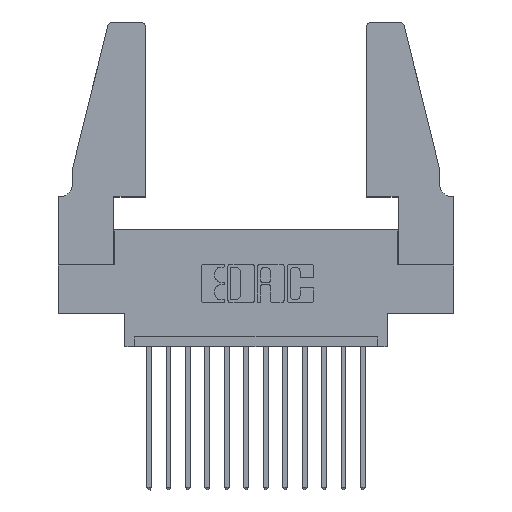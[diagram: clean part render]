
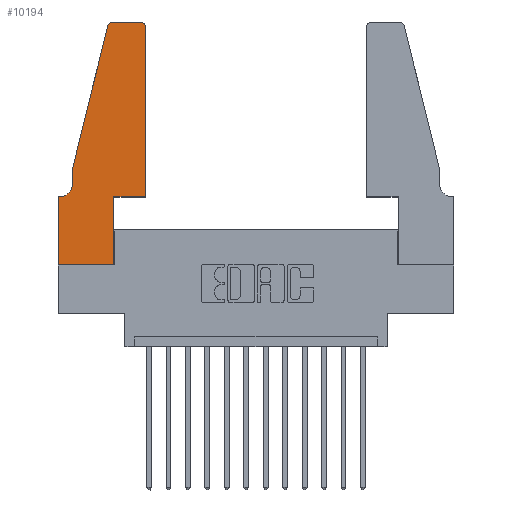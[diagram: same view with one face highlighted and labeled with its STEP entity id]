
A CAD part, top view. The second image highlights one B-rep face of the part: STEP entity #10194.
In plain terms, the highlighted planar face has unit normal (0, 0, 1).
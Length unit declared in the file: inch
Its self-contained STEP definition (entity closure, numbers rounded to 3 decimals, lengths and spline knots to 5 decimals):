
#111 = CARTESIAN_POINT ( 'NONE',  ( 0., 0.35, 0.37 ) ) ;
#120 = ORIENTED_EDGE ( 'NONE', *, *, #9475, .T. ) ;
#334 = CARTESIAN_POINT ( 'NONE',  ( 0., 0.35, 0.37 ) ) ;
#475 = VECTOR ( 'NONE', #14309, 39.37008 ) ;
#499 = EDGE_CURVE ( 'NONE', #13492, #5535, #6857, .T. ) ;
#622 = DIRECTION ( 'NONE',  ( -1., 0., 0. ) ) ;
#713 = DIRECTION ( 'NONE',  ( 1., 0., 0. ) ) ;
#787 = DIRECTION ( 'NONE',  ( 0., 0., -1. ) ) ;
#894 = VERTEX_POINT ( 'NONE', #9341 ) ;
#969 = VERTEX_POINT ( 'NONE', #13915 ) ;
#1103 = DIRECTION ( 'NONE',  ( 0., -1., 0. ) ) ;
#1887 = CARTESIAN_POINT ( 'NONE',  ( 0., 0., 0.37 ) ) ;
#2113 = EDGE_CURVE ( 'NONE', #12750, #4990, #7534, .T. ) ;
#2350 = EDGE_CURVE ( 'NONE', #4990, #13492, #3491, .T. ) ;
#2622 = CIRCLE ( 'NONE', #11793, 0.03 ) ;
#2644 = LINE ( 'NONE', #7715, #12155 ) ;
#2865 = VERTEX_POINT ( 'NONE', #6262 ) ;
#2893 = VECTOR ( 'NONE', #1103, 39.37008 ) ;
#3227 = CARTESIAN_POINT ( 'NONE',  ( 0.4205, 1.22, 0.37 ) ) ;
#3438 = CARTESIAN_POINT ( 'NONE',  ( 0.284, 1.22, 0.37 ) ) ;
#3491 = LINE ( 'NONE', #11873, #475 ) ;
#3603 = CARTESIAN_POINT ( 'NONE',  ( 0.0055, 0.35, 0.37 ) ) ;
#3776 = CARTESIAN_POINT ( 'NONE',  ( 0.4505, 0.35, 0.37 ) ) ;
#4146 = LINE ( 'NONE', #3776, #9891 ) ;
#4171 = AXIS2_PLACEMENT_3D ( 'NONE', #3227, #9069, #5539 ) ;
#4213 = CARTESIAN_POINT ( 'NONE',  ( 0.2605, 1.25, 0.37 ) ) ;
#4229 = DIRECTION ( 'NONE',  ( -1., 0., 0. ) ) ;
#4230 = PLANE ( 'NONE',  #8492 ) ;
#4413 = ORIENTED_EDGE ( 'NONE', *, *, #10837, .T. ) ;
#4791 = CARTESIAN_POINT ( 'NONE',  ( 0.0755, 0.35, 0.37 ) ) ;
#4990 = VERTEX_POINT ( 'NONE', #1887 ) ;
#5039 = ORIENTED_EDGE ( 'NONE', *, *, #499, .T. ) ;
#5523 = CIRCLE ( 'NONE', #14103, 0.07 ) ;
#5535 = VERTEX_POINT ( 'NONE', #12002 ) ;
#5539 = DIRECTION ( 'NONE',  ( 1., 0., 0. ) ) ;
#5576 = VERTEX_POINT ( 'NONE', #3603 ) ;
#5643 = EDGE_CURVE ( 'NONE', #8770, #2865, #2622, .T. ) ;
#5667 = ORIENTED_EDGE ( 'NONE', *, *, #2113, .T. ) ;
#5819 = CARTESIAN_POINT ( 'NONE',  ( 0.284, 1.25, 0.37 ) ) ;
#6110 = VECTOR ( 'NONE', #9176, 39.37008 ) ;
#6180 = CIRCLE ( 'NONE', #4171, 0.03 ) ;
#6262 = CARTESIAN_POINT ( 'NONE',  ( 0.25487, 1.22718, 0.37 ) ) ;
#6572 = CARTESIAN_POINT ( 'NONE',  ( 0.0755, 0.5, 0.37 ) ) ;
#6610 = LINE ( 'NONE', #4213, #7749 ) ;
#6634 = CARTESIAN_POINT ( 'NONE',  ( 0.2865, 0., 0.37 ) ) ;
#6746 = CARTESIAN_POINT ( 'NONE',  ( 0.0755, 0.42, 0.37 ) ) ;
#6857 = LINE ( 'NONE', #8237, #8892 ) ;
#6898 = EDGE_CURVE ( 'NONE', #9258, #8770, #6610, .T. ) ;
#6933 = DIRECTION ( 'NONE',  ( 0., 1., 0. ) ) ;
#7534 = LINE ( 'NONE', #14119, #2893 ) ;
#7715 = CARTESIAN_POINT ( 'NONE',  ( 0.4505, 0.35, 0.37 ) ) ;
#7749 = VECTOR ( 'NONE', #622, 39.37008 ) ;
#7825 = DIRECTION ( 'NONE',  ( 1., 0., 0. ) ) ;
#7851 = LINE ( 'NONE', #4791, #9126 ) ;
#7948 = ORIENTED_EDGE ( 'NONE', *, *, #5643, .T. ) ;
#8216 = FACE_OUTER_BOUND ( 'NONE', #8533, .T. ) ;
#8237 = CARTESIAN_POINT ( 'NONE',  ( 0.2865, 0.35, 0.37 ) ) ;
#8367 = ORIENTED_EDGE ( 'NONE', *, *, #10281, .T. ) ;
#8385 = DIRECTION ( 'NONE',  ( -1., 0., 0. ) ) ;
#8492 = AXIS2_PLACEMENT_3D ( 'NONE', #111, #10684, #13903 ) ;
#8533 = EDGE_LOOP ( 'NONE', ( #9027, #7948, #11964, #4413, #11926, #8367, #5667, #9675, #5039, #120, #15183, #15307 ) ) ;
#8770 = VERTEX_POINT ( 'NONE', #5819 ) ;
#8892 = VECTOR ( 'NONE', #6933, 39.37008 ) ;
#8951 = DIRECTION ( 'NONE',  ( 0., 0., 1. ) ) ;
#9027 = ORIENTED_EDGE ( 'NONE', *, *, #6898, .T. ) ;
#9069 = DIRECTION ( 'NONE',  ( 0., 0., 1. ) ) ;
#9126 = VECTOR ( 'NONE', #8385, 39.37008 ) ;
#9176 = DIRECTION ( 'NONE',  ( -0.239, -0.971, 0. ) ) ;
#9258 = VERTEX_POINT ( 'NONE', #11419 ) ;
#9341 = CARTESIAN_POINT ( 'NONE',  ( 0.4505, 0.35, 0.37 ) ) ;
#9443 = LINE ( 'NONE', #6572, #6110 ) ;
#9475 = EDGE_CURVE ( 'NONE', #5535, #894, #2644, .T. ) ;
#9590 = EDGE_CURVE ( 'NONE', #894, #14440, #4146, .T. ) ;
#9675 = ORIENTED_EDGE ( 'NONE', *, *, #2350, .T. ) ;
#9891 = VECTOR ( 'NONE', #14326, 39.37008 ) ;
#10194 = ADVANCED_FACE ( 'NONE', ( #8216 ), #4230, .T. ) ;
#10281 = EDGE_CURVE ( 'NONE', #5576, #12750, #7851, .T. ) ;
#10684 = DIRECTION ( 'NONE',  ( 0., 0., 1. ) ) ;
#10837 = EDGE_CURVE ( 'NONE', #969, #12025, #15070, .T. ) ;
#11419 = CARTESIAN_POINT ( 'NONE',  ( 0.4205, 1.25, 0.37 ) ) ;
#11793 = AXIS2_PLACEMENT_3D ( 'NONE', #3438, #8951, #713 ) ;
#11873 = CARTESIAN_POINT ( 'NONE',  ( 0., 0., 0.37 ) ) ;
#11926 = ORIENTED_EDGE ( 'NONE', *, *, #12906, .T. ) ;
#11964 = ORIENTED_EDGE ( 'NONE', *, *, #12154, .T. ) ;
#12002 = CARTESIAN_POINT ( 'NONE',  ( 0.2865, 0.35, 0.37 ) ) ;
#12025 = VERTEX_POINT ( 'NONE', #6746 ) ;
#12154 = EDGE_CURVE ( 'NONE', #2865, #969, #9443, .T. ) ;
#12155 = VECTOR ( 'NONE', #7825, 39.37008 ) ;
#12339 = CARTESIAN_POINT ( 'NONE',  ( 0.4505, 1.22, 0.37 ) ) ;
#12750 = VERTEX_POINT ( 'NONE', #334 ) ;
#12906 = EDGE_CURVE ( 'NONE', #12025, #5576, #5523, .T. ) ;
#13492 = VERTEX_POINT ( 'NONE', #6634 ) ;
#13903 = DIRECTION ( 'NONE',  ( 1., 0., 0. ) ) ;
#13915 = CARTESIAN_POINT ( 'NONE',  ( 0.0755, 0.5, 0.37 ) ) ;
#13962 = VECTOR ( 'NONE', #14896, 39.37008 ) ;
#14103 = AXIS2_PLACEMENT_3D ( 'NONE', #14978, #787, #4229 ) ;
#14119 = CARTESIAN_POINT ( 'NONE',  ( 0., 0., 0.37 ) ) ;
#14309 = DIRECTION ( 'NONE',  ( 1., 0., 0. ) ) ;
#14326 = DIRECTION ( 'NONE',  ( 0., 1., 0. ) ) ;
#14440 = VERTEX_POINT ( 'NONE', #12339 ) ;
#14799 = CARTESIAN_POINT ( 'NONE',  ( 0.0755, 0.5, 0.37 ) ) ;
#14896 = DIRECTION ( 'NONE',  ( 0., -1., 0. ) ) ;
#14978 = CARTESIAN_POINT ( 'NONE',  ( 0.0055, 0.42, 0.37 ) ) ;
#15070 = LINE ( 'NONE', #14799, #13962 ) ;
#15183 = ORIENTED_EDGE ( 'NONE', *, *, #9590, .T. ) ;
#15275 = EDGE_CURVE ( 'NONE', #14440, #9258, #6180, .T. ) ;
#15307 = ORIENTED_EDGE ( 'NONE', *, *, #15275, .T. ) ;
